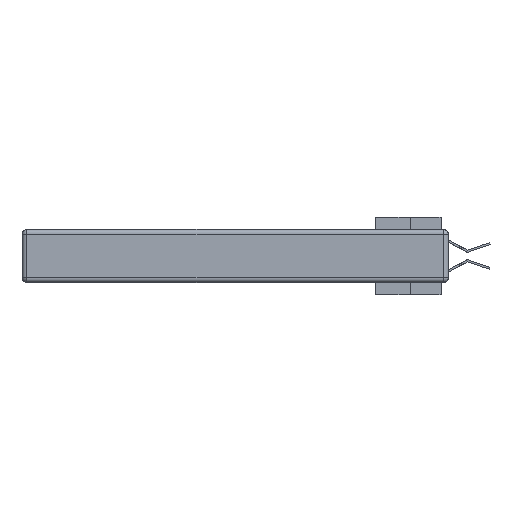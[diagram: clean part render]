
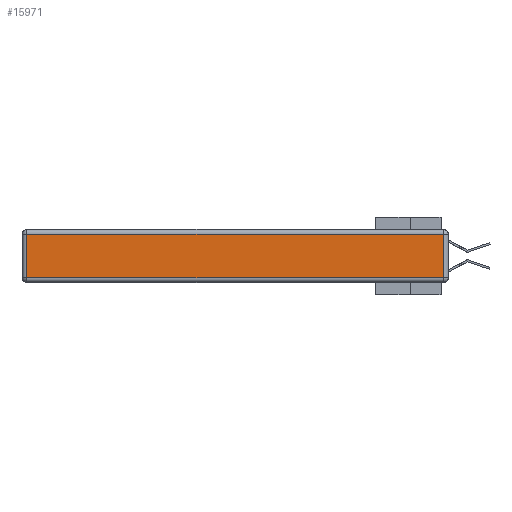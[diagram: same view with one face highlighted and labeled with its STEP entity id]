
A CAD part, left-side view. The second image highlights one B-rep face of the part: STEP entity #15971.
In plain terms, the highlighted planar face has unit normal (-1, 0, 0).
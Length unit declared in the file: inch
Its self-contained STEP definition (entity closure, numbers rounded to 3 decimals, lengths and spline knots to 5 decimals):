
#297 = DIRECTION ( 'NONE',  ( 0., 0., 1. ) ) ;
#596 = DIRECTION ( 'NONE',  ( 0., 0., -1. ) ) ;
#1065 = CARTESIAN_POINT ( 'NONE',  ( 0., 0., -0.313 ) ) ;
#2831 = LINE ( 'NONE', #24975, #33599 ) ;
#3527 = VERTEX_POINT ( 'NONE', #36402 ) ;
#4526 = CARTESIAN_POINT ( 'NONE',  ( 0., 2.72, -0.313 ) ) ;
#6483 = CARTESIAN_POINT ( 'NONE',  ( 0., 0.03, -0.03 ) ) ;
#7515 = DIRECTION ( 'NONE',  ( 0., -1., 0. ) ) ;
#7919 = LINE ( 'NONE', #29735, #13427 ) ;
#11571 = VERTEX_POINT ( 'NONE', #4526 ) ;
#12402 = VECTOR ( 'NONE', #7515, 39.37008 ) ;
#13427 = VECTOR ( 'NONE', #596, 39.37008 ) ;
#13560 = DIRECTION ( 'NONE',  ( -1., 0., 0. ) ) ;
#13593 = AXIS2_PLACEMENT_3D ( 'NONE', #32734, #13560, #297 ) ;
#15971 = ADVANCED_FACE ( 'NONE', ( #22194 ), #38987, .T. ) ;
#18580 = EDGE_LOOP ( 'NONE', ( #41376, #28937, #35000, #32102 ) ) ;
#18608 = VERTEX_POINT ( 'NONE', #6483 ) ;
#20643 = EDGE_CURVE ( 'NONE', #3527, #18608, #26451, .T. ) ;
#22154 = DIRECTION ( 'NONE',  ( 0., 1., 0. ) ) ;
#22194 = FACE_OUTER_BOUND ( 'NONE', #18580, .T. ) ;
#22910 = DIRECTION ( 'NONE',  ( 0., 0., 1. ) ) ;
#24850 = VERTEX_POINT ( 'NONE', #27233 ) ;
#24975 = CARTESIAN_POINT ( 'NONE',  ( 0., 2.75, -0.03 ) ) ;
#26451 = LINE ( 'NONE', #29293, #29976 ) ;
#27233 = CARTESIAN_POINT ( 'NONE',  ( 0., 2.72, -0.03 ) ) ;
#28937 = ORIENTED_EDGE ( 'NONE', *, *, #20643, .T. ) ;
#29293 = CARTESIAN_POINT ( 'NONE',  ( 0., 0.03, -0.343 ) ) ;
#29735 = CARTESIAN_POINT ( 'NONE',  ( 0., 2.72, -0.343 ) ) ;
#29976 = VECTOR ( 'NONE', #22910, 39.37008 ) ;
#31954 = EDGE_CURVE ( 'NONE', #18608, #24850, #2831, .T. ) ;
#32102 = ORIENTED_EDGE ( 'NONE', *, *, #39064, .T. ) ;
#32734 = CARTESIAN_POINT ( 'NONE',  ( 0., 0., -0.343 ) ) ;
#33599 = VECTOR ( 'NONE', #22154, 39.37008 ) ;
#33680 = EDGE_CURVE ( 'NONE', #11571, #3527, #36923, .T. ) ;
#35000 = ORIENTED_EDGE ( 'NONE', *, *, #31954, .T. ) ;
#36402 = CARTESIAN_POINT ( 'NONE',  ( 0., 0.03, -0.313 ) ) ;
#36923 = LINE ( 'NONE', #1065, #12402 ) ;
#38987 = PLANE ( 'NONE',  #13593 ) ;
#39064 = EDGE_CURVE ( 'NONE', #24850, #11571, #7919, .T. ) ;
#41376 = ORIENTED_EDGE ( 'NONE', *, *, #33680, .T. ) ;
